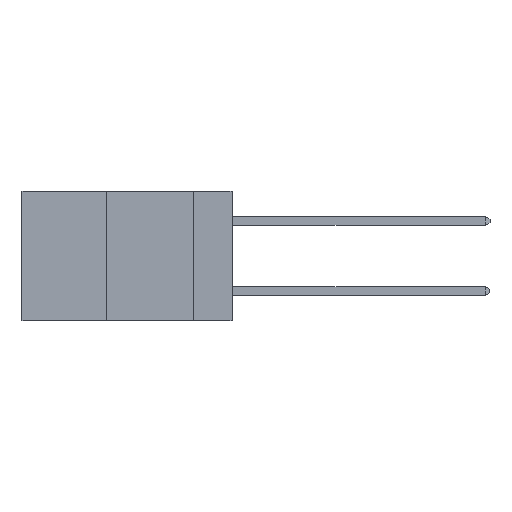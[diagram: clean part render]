
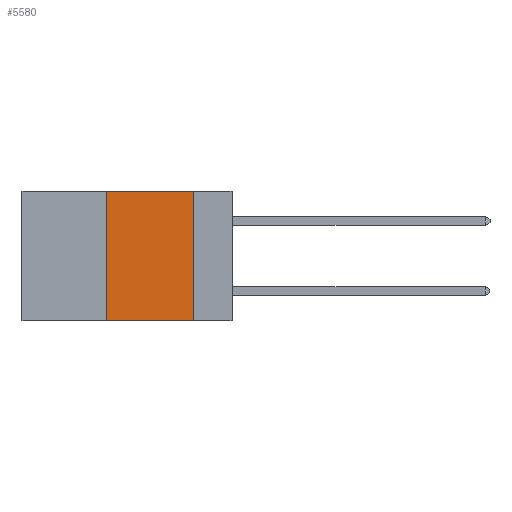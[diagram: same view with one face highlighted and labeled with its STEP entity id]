
A CAD part, left-side view. The second image highlights one B-rep face of the part: STEP entity #5580.
In plain terms, the highlighted planar face has unit normal (-1, 0, 0).
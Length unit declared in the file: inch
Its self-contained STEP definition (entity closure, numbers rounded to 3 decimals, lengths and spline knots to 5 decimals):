
#199 = EDGE_LOOP ( 'NONE', ( #9230, #17771, #7445, #17547 ) ) ;
#202 = VECTOR ( 'NONE', #19933, 39.37008 ) ;
#1207 = CARTESIAN_POINT ( 'NONE',  ( 0., 0.6, 0. ) ) ;
#2019 = DIRECTION ( 'NONE',  ( 0., -1., 0. ) ) ;
#4794 = EDGE_CURVE ( 'NONE', #11987, #8085, #4836, .T. ) ;
#4836 = LINE ( 'NONE', #18349, #202 ) ;
#5580 = ADVANCED_FACE ( 'NONE', ( #11078 ), #7897, .F. ) ;
#6362 = DIRECTION ( 'NONE',  ( 1., 0., 0. ) ) ;
#6718 = VECTOR ( 'NONE', #2019, 39.37008 ) ;
#7047 = CARTESIAN_POINT ( 'NONE',  ( 0., 0.6, -0.37 ) ) ;
#7445 = ORIENTED_EDGE ( 'NONE', *, *, #15975, .F. ) ;
#7813 = VECTOR ( 'NONE', #20666, 39.37008 ) ;
#7897 = PLANE ( 'NONE',  #13592 ) ;
#8085 = VERTEX_POINT ( 'NONE', #20484 ) ;
#8830 = VERTEX_POINT ( 'NONE', #15042 ) ;
#9230 = ORIENTED_EDGE ( 'NONE', *, *, #4794, .F. ) ;
#11078 = FACE_OUTER_BOUND ( 'NONE', #199, .T. ) ;
#11339 = VECTOR ( 'NONE', #15399, 39.37008 ) ;
#11577 = CARTESIAN_POINT ( 'NONE',  ( 0., 0.11, 0. ) ) ;
#11987 = VERTEX_POINT ( 'NONE', #11577 ) ;
#12116 = LINE ( 'NONE', #14315, #7813 ) ;
#12289 = VERTEX_POINT ( 'NONE', #17198 ) ;
#12729 = EDGE_CURVE ( 'NONE', #12289, #8085, #20494, .T. ) ;
#13592 = AXIS2_PLACEMENT_3D ( 'NONE', #1207, #6362, #17618 ) ;
#14315 = CARTESIAN_POINT ( 'NONE',  ( 0., 0.36, 0. ) ) ;
#15042 = CARTESIAN_POINT ( 'NONE',  ( 0., 0.36, 0. ) ) ;
#15399 = DIRECTION ( 'NONE',  ( 0., -1., 0. ) ) ;
#15640 = LINE ( 'NONE', #17019, #11339 ) ;
#15753 = EDGE_CURVE ( 'NONE', #8830, #11987, #15640, .T. ) ;
#15975 = EDGE_CURVE ( 'NONE', #12289, #8830, #12116, .T. ) ;
#17019 = CARTESIAN_POINT ( 'NONE',  ( 0., 0.6, 0. ) ) ;
#17198 = CARTESIAN_POINT ( 'NONE',  ( 0., 0.36, -0.37 ) ) ;
#17547 = ORIENTED_EDGE ( 'NONE', *, *, #12729, .T. ) ;
#17618 = DIRECTION ( 'NONE',  ( 0., 0., -1. ) ) ;
#17771 = ORIENTED_EDGE ( 'NONE', *, *, #15753, .F. ) ;
#18349 = CARTESIAN_POINT ( 'NONE',  ( 0., 0.11, 0. ) ) ;
#19933 = DIRECTION ( 'NONE',  ( 0., 0., -1. ) ) ;
#20484 = CARTESIAN_POINT ( 'NONE',  ( 0., 0.11, -0.37 ) ) ;
#20494 = LINE ( 'NONE', #7047, #6718 ) ;
#20666 = DIRECTION ( 'NONE',  ( 0., 0., 1. ) ) ;
